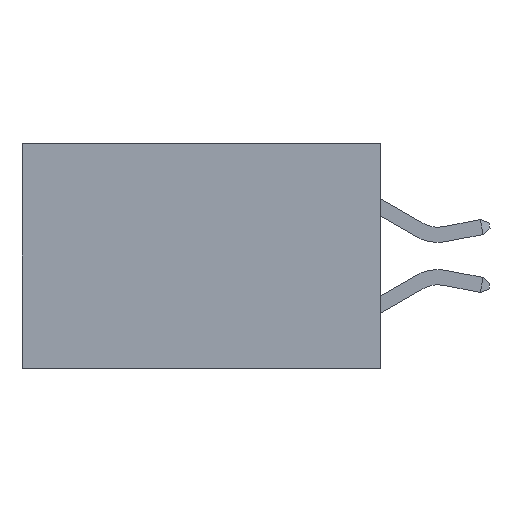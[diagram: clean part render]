
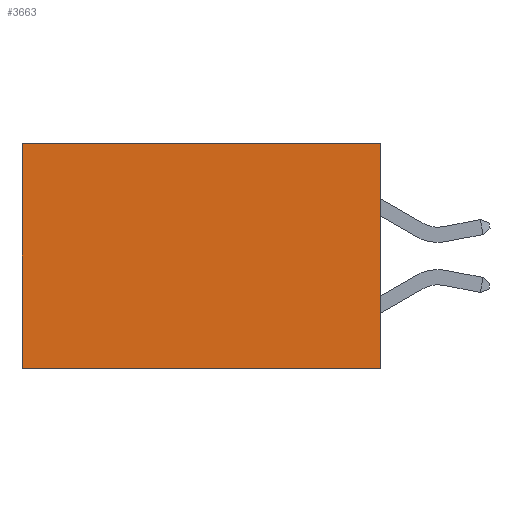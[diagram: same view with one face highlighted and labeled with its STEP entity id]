
A CAD part, left-side view. The second image highlights one B-rep face of the part: STEP entity #3663.
In plain terms, the highlighted planar face has unit normal (-1, 0, 0).
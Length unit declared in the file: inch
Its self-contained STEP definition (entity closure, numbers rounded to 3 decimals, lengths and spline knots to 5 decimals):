
#28 = EDGE_CURVE ( 'NONE', #2083, #58, #2148, .T. ) ;
#58 = VERTEX_POINT ( 'NONE', #6403 ) ;
#116 = DIRECTION ( 'NONE',  ( 0., 1., 0. ) ) ;
#308 = VERTEX_POINT ( 'NONE', #388 ) ;
#388 = CARTESIAN_POINT ( 'NONE',  ( 0.277, 0.59, 0. ) ) ;
#410 = VERTEX_POINT ( 'NONE', #3564 ) ;
#430 = LINE ( 'NONE', #3828, #7061 ) ;
#477 = EDGE_CURVE ( 'NONE', #308, #58, #1924, .T. ) ;
#1129 = LINE ( 'NONE', #2222, #7645 ) ;
#1170 = ORIENTED_EDGE ( 'NONE', *, *, #28, .F. ) ;
#1924 = LINE ( 'NONE', #7498, #3486 ) ;
#2083 = VERTEX_POINT ( 'NONE', #4615 ) ;
#2148 = LINE ( 'NONE', #4299, #5338 ) ;
#2222 = CARTESIAN_POINT ( 'NONE',  ( 0.277, 0., 0. ) ) ;
#2889 = DIRECTION ( 'NONE',  ( 0., 1., 0. ) ) ;
#3160 = DIRECTION ( 'NONE',  ( 0., 0., -1. ) ) ;
#3486 = VECTOR ( 'NONE', #3160, 39.37008 ) ;
#3564 = CARTESIAN_POINT ( 'NONE',  ( 0.277, 0., 0. ) ) ;
#3590 = EDGE_LOOP ( 'NONE', ( #7914, #1170, #6932, #6107 ) ) ;
#3663 = ADVANCED_FACE ( 'NONE', ( #5966 ), #4688, .F. ) ;
#3828 = CARTESIAN_POINT ( 'NONE',  ( 0.277, 0., -0.37 ) ) ;
#3875 = DIRECTION ( 'NONE',  ( 0., 0., -1. ) ) ;
#4232 = EDGE_CURVE ( 'NONE', #410, #2083, #430, .T. ) ;
#4268 = AXIS2_PLACEMENT_3D ( 'NONE', #4632, #4681, #4667 ) ;
#4299 = CARTESIAN_POINT ( 'NONE',  ( 0.277, 0., -0.37 ) ) ;
#4615 = CARTESIAN_POINT ( 'NONE',  ( 0.277, 0., -0.37 ) ) ;
#4632 = CARTESIAN_POINT ( 'NONE',  ( 0.277, 0., -0.37 ) ) ;
#4667 = DIRECTION ( 'NONE',  ( 0., 0., -1. ) ) ;
#4681 = DIRECTION ( 'NONE',  ( 1., 0., 0. ) ) ;
#4688 = PLANE ( 'NONE',  #4268 ) ;
#5338 = VECTOR ( 'NONE', #116, 39.37008 ) ;
#5966 = FACE_OUTER_BOUND ( 'NONE', #3590, .T. ) ;
#6107 = ORIENTED_EDGE ( 'NONE', *, *, #7993, .T. ) ;
#6403 = CARTESIAN_POINT ( 'NONE',  ( 0.277, 0.59, -0.37 ) ) ;
#6932 = ORIENTED_EDGE ( 'NONE', *, *, #4232, .F. ) ;
#7061 = VECTOR ( 'NONE', #3875, 39.37008 ) ;
#7498 = CARTESIAN_POINT ( 'NONE',  ( 0.277, 0.59, -0.37 ) ) ;
#7645 = VECTOR ( 'NONE', #2889, 39.37008 ) ;
#7914 = ORIENTED_EDGE ( 'NONE', *, *, #477, .T. ) ;
#7993 = EDGE_CURVE ( 'NONE', #410, #308, #1129, .T. ) ;
